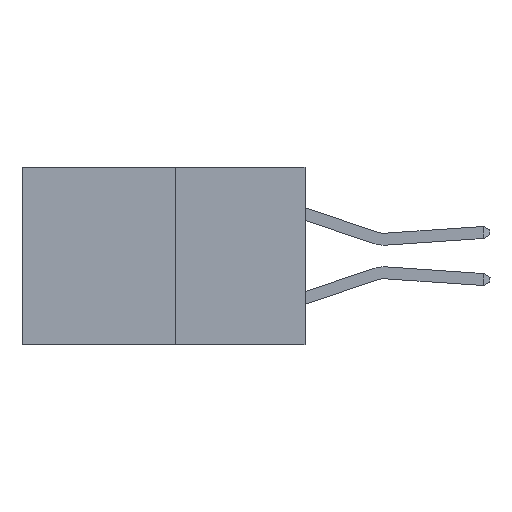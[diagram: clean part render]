
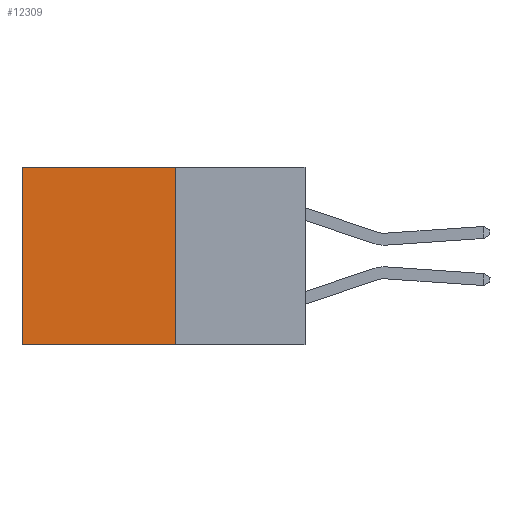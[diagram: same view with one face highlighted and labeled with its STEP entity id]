
A CAD part, left-side view. The second image highlights one B-rep face of the part: STEP entity #12309.
In plain terms, the highlighted planar face has unit normal (-1, 0, 0).
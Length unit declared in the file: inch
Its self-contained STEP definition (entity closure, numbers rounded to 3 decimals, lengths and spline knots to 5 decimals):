
#1736 = LINE ( 'NONE', #15473, #20522 ) ;
#1835 = VERTEX_POINT ( 'NONE', #7222 ) ;
#2117 = LINE ( 'NONE', #15254, #20900 ) ;
#2324 = VERTEX_POINT ( 'NONE', #13207 ) ;
#2789 = EDGE_CURVE ( 'NONE', #1835, #2324, #2117, .T. ) ;
#3908 = CARTESIAN_POINT ( 'NONE',  ( 0.277, 0.59, 0. ) ) ;
#5173 = VECTOR ( 'NONE', #23316, 39.37008 ) ;
#5494 = DIRECTION ( 'NONE',  ( 0., 1., 0. ) ) ;
#5903 = EDGE_LOOP ( 'NONE', ( #20650, #12295, #7931, #17909 ) ) ;
#6526 = DIRECTION ( 'NONE',  ( 0., 0., -1. ) ) ;
#7222 = CARTESIAN_POINT ( 'NONE',  ( 0.277, 0.27, 0. ) ) ;
#7931 = ORIENTED_EDGE ( 'NONE', *, *, #2789, .F. ) ;
#9158 = CARTESIAN_POINT ( 'NONE',  ( 0.277, 0.27, 0. ) ) ;
#10620 = DIRECTION ( 'NONE',  ( 0., 0., -1. ) ) ;
#12024 = DIRECTION ( 'NONE',  ( 0., 0., -1. ) ) ;
#12295 = ORIENTED_EDGE ( 'NONE', *, *, #15120, .F. ) ;
#12309 = ADVANCED_FACE ( 'NONE', ( #16650 ), #21053, .F. ) ;
#13207 = CARTESIAN_POINT ( 'NONE',  ( 0.277, 0.27, -0.37 ) ) ;
#14477 = AXIS2_PLACEMENT_3D ( 'NONE', #17414, #22863, #12024 ) ;
#15120 = EDGE_CURVE ( 'NONE', #2324, #19070, #20206, .T. ) ;
#15254 = CARTESIAN_POINT ( 'NONE',  ( 0.277, 0.27, -0.37 ) ) ;
#15473 = CARTESIAN_POINT ( 'NONE',  ( 0.277, 0.59, -0.37 ) ) ;
#16650 = FACE_OUTER_BOUND ( 'NONE', #5903, .T. ) ;
#16865 = EDGE_CURVE ( 'NONE', #1835, #23310, #18895, .T. ) ;
#17414 = CARTESIAN_POINT ( 'NONE',  ( 0.277, 0.27, -0.37 ) ) ;
#17909 = ORIENTED_EDGE ( 'NONE', *, *, #16865, .T. ) ;
#17944 = CARTESIAN_POINT ( 'NONE',  ( 0.277, 0.27, -0.37 ) ) ;
#18029 = CARTESIAN_POINT ( 'NONE',  ( 0.277, 0.59, -0.37 ) ) ;
#18895 = LINE ( 'NONE', #9158, #23151 ) ;
#19070 = VERTEX_POINT ( 'NONE', #18029 ) ;
#20206 = LINE ( 'NONE', #17944, #5173 ) ;
#20522 = VECTOR ( 'NONE', #6526, 39.37008 ) ;
#20650 = ORIENTED_EDGE ( 'NONE', *, *, #22851, .T. ) ;
#20900 = VECTOR ( 'NONE', #10620, 39.37008 ) ;
#21053 = PLANE ( 'NONE',  #14477 ) ;
#22851 = EDGE_CURVE ( 'NONE', #23310, #19070, #1736, .T. ) ;
#22863 = DIRECTION ( 'NONE',  ( 1., 0., 0. ) ) ;
#23151 = VECTOR ( 'NONE', #5494, 39.37008 ) ;
#23310 = VERTEX_POINT ( 'NONE', #3908 ) ;
#23316 = DIRECTION ( 'NONE',  ( 0., 1., 0. ) ) ;
